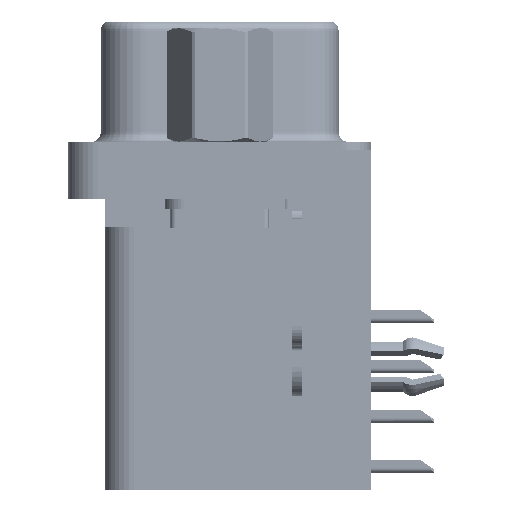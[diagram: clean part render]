
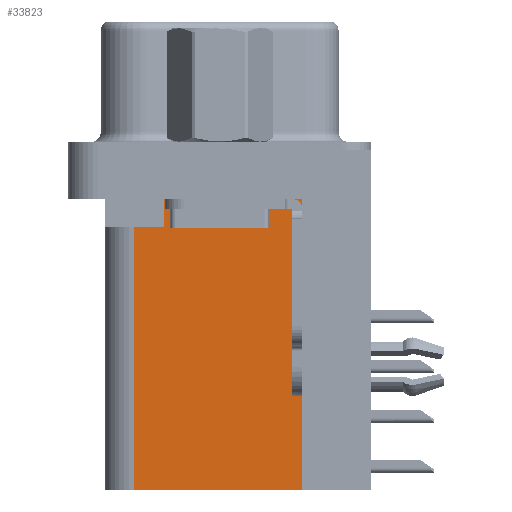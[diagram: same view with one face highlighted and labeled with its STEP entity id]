
A CAD part, left-side view. The second image highlights one B-rep face of the part: STEP entity #33823.
In plain terms, the highlighted planar face has unit normal (-1, 0, 0).
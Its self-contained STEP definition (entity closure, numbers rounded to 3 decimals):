
#1185 = CARTESIAN_POINT ( 'NONE',  ( 3.75, 4.35, -17.3 ) ) ;
#1432 = DIRECTION ( 'NONE',  ( 0., 0., -1. ) ) ;
#2692 = LINE ( 'NONE', #9302, #21059 ) ;
#2944 = AXIS2_PLACEMENT_3D ( 'NONE', #32638, #18031, #43855 ) ;
#3096 = ORIENTED_EDGE ( 'NONE', *, *, #21781, .T. ) ;
#3434 = DIRECTION ( 'NONE',  ( 0., 1., 0. ) ) ;
#4413 = CARTESIAN_POINT ( 'NONE',  ( 3.75, 2.85, -2.5 ) ) ;
#4577 = CARTESIAN_POINT ( 'NONE',  ( 3.75, -4.2, -2.5 ) ) ;
#4936 = DIRECTION ( 'NONE',  ( 0., 0., 1. ) ) ;
#6446 = DIRECTION ( 'NONE',  ( 0., 1., 0. ) ) ;
#6487 = ORIENTED_EDGE ( 'NONE', *, *, #13565, .T. ) ;
#7105 = CARTESIAN_POINT ( 'NONE',  ( 3.75, 4.35, -17.3 ) ) ;
#7130 = ORIENTED_EDGE ( 'NONE', *, *, #31374, .F. ) ;
#9302 = CARTESIAN_POINT ( 'NONE',  ( 3.75, -4.2, -17.3 ) ) ;
#9828 = VECTOR ( 'NONE', #39059, 1000. ) ;
#10494 = EDGE_CURVE ( 'NONE', #37505, #43917, #25184, .T. ) ;
#10645 = CARTESIAN_POINT ( 'NONE',  ( 3.75, -4.2, -2.5 ) ) ;
#12946 = DIRECTION ( 'NONE',  ( 0., 0., 1. ) ) ;
#13565 = EDGE_CURVE ( 'NONE', #31279, #43917, #21827, .T. ) ;
#14962 = ORIENTED_EDGE ( 'NONE', *, *, #10494, .F. ) ;
#15456 = FACE_OUTER_BOUND ( 'NONE', #43826, .T. ) ;
#16190 = CARTESIAN_POINT ( 'NONE',  ( 3.75, 2.85, -3.9 ) ) ;
#17314 = VECTOR ( 'NONE', #1432, 1000. ) ;
#18031 = DIRECTION ( 'NONE',  ( 1., 0., 0. ) ) ;
#18128 = LINE ( 'NONE', #10645, #36584 ) ;
#19974 = VERTEX_POINT ( 'NONE', #4413 ) ;
#20599 = VECTOR ( 'NONE', #4936, 1000. ) ;
#21059 = VECTOR ( 'NONE', #12946, 1000. ) ;
#21781 = EDGE_CURVE ( 'NONE', #39654, #19974, #18128, .T. ) ;
#21827 = LINE ( 'NONE', #42598, #9828 ) ;
#23307 = CARTESIAN_POINT ( 'NONE',  ( 3.75, -4.2, -17.3 ) ) ;
#23499 = CARTESIAN_POINT ( 'NONE',  ( 3.75, 4.35, -3.9 ) ) ;
#24188 = LINE ( 'NONE', #46876, #43911 ) ;
#25184 = LINE ( 'NONE', #1185, #20599 ) ;
#27026 = LINE ( 'NONE', #16190, #17314 ) ;
#28391 = ORIENTED_EDGE ( 'NONE', *, *, #40532, .T. ) ;
#31279 = VERTEX_POINT ( 'NONE', #46401 ) ;
#31374 = EDGE_CURVE ( 'NONE', #41103, #37505, #24188, .T. ) ;
#32638 = CARTESIAN_POINT ( 'NONE',  ( 3.75, -4.2, -17.3 ) ) ;
#33823 = ADVANCED_FACE ( 'NONE', ( #15456 ), #40186, .F. ) ;
#36584 = VECTOR ( 'NONE', #3434, 1000. ) ;
#37505 = VERTEX_POINT ( 'NONE', #7105 ) ;
#39059 = DIRECTION ( 'NONE',  ( 0., 1., 0. ) ) ;
#39654 = VERTEX_POINT ( 'NONE', #4577 ) ;
#40186 = PLANE ( 'NONE',  #2944 ) ;
#40532 = EDGE_CURVE ( 'NONE', #41103, #39654, #2692, .T. ) ;
#41103 = VERTEX_POINT ( 'NONE', #23307 ) ;
#42598 = CARTESIAN_POINT ( 'NONE',  ( 3.75, 0., -3.9 ) ) ;
#43826 = EDGE_LOOP ( 'NONE', ( #3096, #46926, #6487, #14962, #7130, #28391 ) ) ;
#43855 = DIRECTION ( 'NONE',  ( 0., 1., 0. ) ) ;
#43911 = VECTOR ( 'NONE', #6446, 1000. ) ;
#43917 = VERTEX_POINT ( 'NONE', #23499 ) ;
#44666 = EDGE_CURVE ( 'NONE', #19974, #31279, #27026, .T. ) ;
#46401 = CARTESIAN_POINT ( 'NONE',  ( 3.75, 2.85, -3.9 ) ) ;
#46876 = CARTESIAN_POINT ( 'NONE',  ( 3.75, -4.2, -17.3 ) ) ;
#46926 = ORIENTED_EDGE ( 'NONE', *, *, #44666, .T. ) ;
